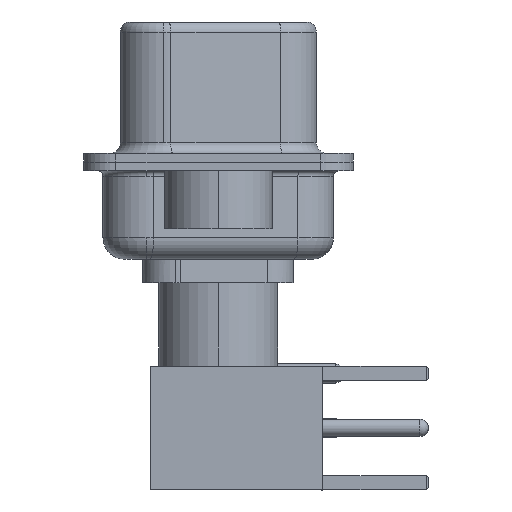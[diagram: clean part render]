
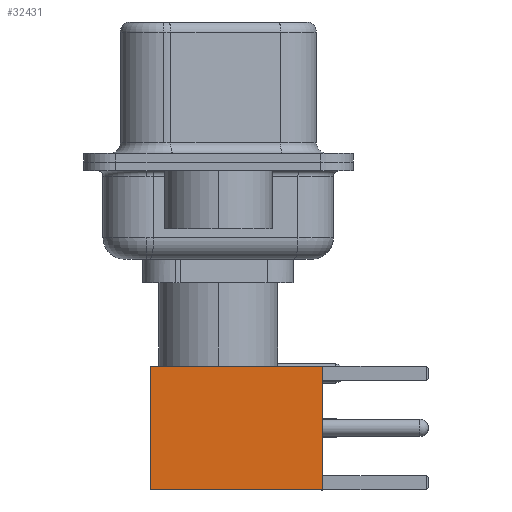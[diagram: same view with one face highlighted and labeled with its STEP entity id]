
A CAD part, left-side view. The second image highlights one B-rep face of the part: STEP entity #32431.
In plain terms, the highlighted face is planar.
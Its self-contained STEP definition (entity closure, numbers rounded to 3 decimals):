
#1701 = AXIS2_PLACEMENT_3D ( 'NONE', #18816, #28950, #2870 ) ;
#1864 = LINE ( 'NONE', #27131, #16995 ) ;
#2590 = DIRECTION ( 'NONE',  ( 0., 0., -1. ) ) ;
#2870 = DIRECTION ( 'NONE',  ( 0., 0., 1. ) ) ;
#3156 = EDGE_CURVE ( 'NONE', #21158, #17192, #6170, .T. ) ;
#5091 = CARTESIAN_POINT ( 'NONE',  ( 2.875, 2.875, 8. ) ) ;
#6170 = LINE ( 'NONE', #26127, #15545 ) ;
#6338 = DIRECTION ( 'NONE',  ( -1., 0., 0. ) ) ;
#6518 = VERTEX_POINT ( 'NONE', #5091 ) ;
#6521 = ORIENTED_EDGE ( 'NONE', *, *, #3156, .T. ) ;
#6793 = CARTESIAN_POINT ( 'NONE',  ( 2.875, 2.875, 0. ) ) ;
#7133 = CARTESIAN_POINT ( 'NONE',  ( -2.875, 2.875, 8. ) ) ;
#8642 = ORIENTED_EDGE ( 'NONE', *, *, #15207, .F. ) ;
#10750 = CARTESIAN_POINT ( 'NONE',  ( 2.875, 2.875, 0. ) ) ;
#11171 = PLANE ( 'NONE',  #1701 ) ;
#12018 = DIRECTION ( 'NONE',  ( -1., 0., 0. ) ) ;
#13203 = EDGE_CURVE ( 'NONE', #6518, #21158, #20385, .T. ) ;
#15072 = DIRECTION ( 'NONE',  ( 0., 0., -1. ) ) ;
#15207 = EDGE_CURVE ( 'NONE', #24375, #17192, #25039, .T. ) ;
#15545 = VECTOR ( 'NONE', #6338, 1000. ) ;
#16729 = ORIENTED_EDGE ( 'NONE', *, *, #13203, .T. ) ;
#16995 = VECTOR ( 'NONE', #12018, 1000. ) ;
#17060 = EDGE_LOOP ( 'NONE', ( #16729, #6521, #8642, #25315 ) ) ;
#17192 = VERTEX_POINT ( 'NONE', #24200 ) ;
#18816 = CARTESIAN_POINT ( 'NONE',  ( 2.875, 2.875, 0. ) ) ;
#20385 = LINE ( 'NONE', #10750, #22267 ) ;
#21158 = VERTEX_POINT ( 'NONE', #6793 ) ;
#22267 = VECTOR ( 'NONE', #2590, 1000. ) ;
#22559 = CARTESIAN_POINT ( 'NONE',  ( -2.875, 2.875, 0. ) ) ;
#23928 = EDGE_CURVE ( 'NONE', #6518, #24375, #1864, .T. ) ;
#24200 = CARTESIAN_POINT ( 'NONE',  ( -2.875, 2.875, 0. ) ) ;
#24375 = VERTEX_POINT ( 'NONE', #7133 ) ;
#25039 = LINE ( 'NONE', #22559, #27569 ) ;
#25315 = ORIENTED_EDGE ( 'NONE', *, *, #23928, .F. ) ;
#26127 = CARTESIAN_POINT ( 'NONE',  ( 0., 2.875, 0. ) ) ;
#27131 = CARTESIAN_POINT ( 'NONE',  ( 0., 2.875, 8. ) ) ;
#27569 = VECTOR ( 'NONE', #15072, 1000. ) ;
#28950 = DIRECTION ( 'NONE',  ( 0., 1., 0. ) ) ;
#31437 = FACE_OUTER_BOUND ( 'NONE', #17060, .T. ) ;
#32431 = ADVANCED_FACE ( 'NONE', ( #31437 ), #11171, .T. ) ;
